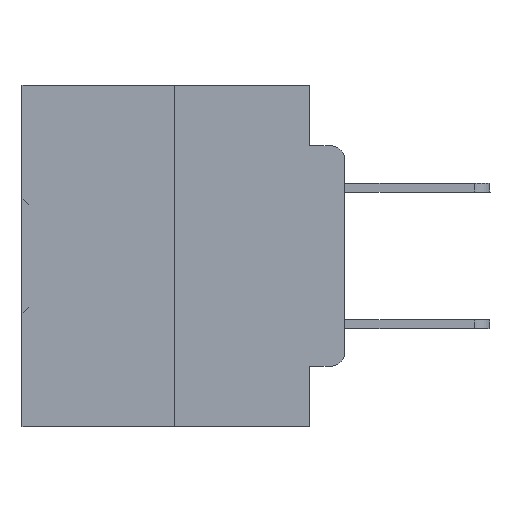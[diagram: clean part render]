
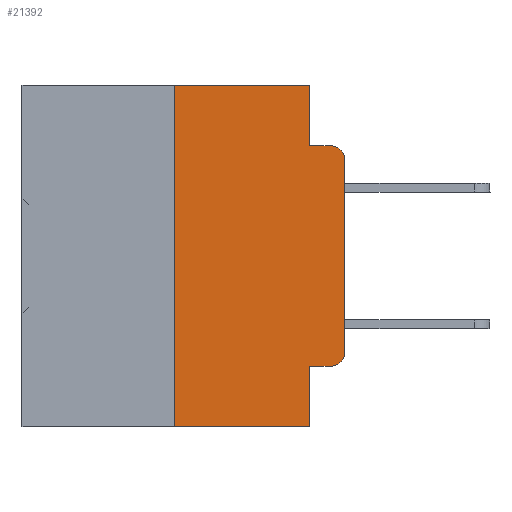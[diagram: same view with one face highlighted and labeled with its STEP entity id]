
A CAD part, left-side view. The second image highlights one B-rep face of the part: STEP entity #21392.
In plain terms, the highlighted planar face has unit normal (-1, 0, 0).
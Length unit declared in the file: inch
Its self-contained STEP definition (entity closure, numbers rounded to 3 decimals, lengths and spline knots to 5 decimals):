
#1253 = AXIS2_PLACEMENT_3D ( 'NONE', #6775, #26557, #9620 ) ;
#1346 = ORIENTED_EDGE ( 'NONE', *, *, #23523, .F. ) ;
#1879 = CARTESIAN_POINT ( 'NONE',  ( 0., 0.051, -0.4115 ) ) ;
#2084 = DIRECTION ( 'NONE',  ( 0., 0., -1. ) ) ;
#2875 = VECTOR ( 'NONE', #15385, 39.37008 ) ;
#3985 = CARTESIAN_POINT ( 'NONE',  ( 0., 0.051, 0. ) ) ;
#4234 = DIRECTION ( 'NONE',  ( 0., 0., 1. ) ) ;
#4539 = VERTEX_POINT ( 'NONE', #21378 ) ;
#4730 = CARTESIAN_POINT ( 'NONE',  ( 0., 0.25, -0.5 ) ) ;
#4980 = ORIENTED_EDGE ( 'NONE', *, *, #17506, .T. ) ;
#5742 = VECTOR ( 'NONE', #13150, 39.37008 ) ;
#6094 = VERTEX_POINT ( 'NONE', #4730 ) ;
#6095 = VECTOR ( 'NONE', #30946, 39.37008 ) ;
#6140 = DIRECTION ( 'NONE',  ( 0., 0., -1. ) ) ;
#6775 = CARTESIAN_POINT ( 'NONE',  ( 0., 0.02, -0.1085 ) ) ;
#7444 = CARTESIAN_POINT ( 'NONE',  ( 0., 0.051, -0.4115 ) ) ;
#7494 = CARTESIAN_POINT ( 'NONE',  ( 0., 0.473, -0.5 ) ) ;
#9620 = DIRECTION ( 'NONE',  ( 0., 0., -1. ) ) ;
#9769 = CARTESIAN_POINT ( 'NONE',  ( 0., 0.051, 0. ) ) ;
#10288 = ORIENTED_EDGE ( 'NONE', *, *, #15849, .T. ) ;
#10762 = ORIENTED_EDGE ( 'NONE', *, *, #18948, .F. ) ;
#11372 = AXIS2_PLACEMENT_3D ( 'NONE', #31407, #23121, #6140 ) ;
#11918 = AXIS2_PLACEMENT_3D ( 'NONE', #35868, #19095, #2084 ) ;
#11961 = VERTEX_POINT ( 'NONE', #1879 ) ;
#12064 = CARTESIAN_POINT ( 'NONE',  ( 0., 0., -0.3915 ) ) ;
#13150 = DIRECTION ( 'NONE',  ( 0., -1., 0. ) ) ;
#13276 = LINE ( 'NONE', #7444, #5742 ) ;
#13991 = EDGE_CURVE ( 'NONE', #31617, #19592, #15132, .T. ) ;
#14046 = CARTESIAN_POINT ( 'NONE',  ( 0., 0., 0. ) ) ;
#14082 = ORIENTED_EDGE ( 'NONE', *, *, #17052, .T. ) ;
#14471 = LINE ( 'NONE', #14046, #6095 ) ;
#14996 = CARTESIAN_POINT ( 'NONE',  ( 0., 0.02, -0.4115 ) ) ;
#15009 = LINE ( 'NONE', #24076, #36550 ) ;
#15132 = CIRCLE ( 'NONE', #11918, 0.02 ) ;
#15305 = LINE ( 'NONE', #7494, #30333 ) ;
#15385 = DIRECTION ( 'NONE',  ( 0., 0., -1. ) ) ;
#15725 = VERTEX_POINT ( 'NONE', #32226 ) ;
#15775 = VERTEX_POINT ( 'NONE', #35252 ) ;
#15849 = EDGE_CURVE ( 'NONE', #11961, #31617, #13276, .T. ) ;
#16867 = ORIENTED_EDGE ( 'NONE', *, *, #19712, .F. ) ;
#16913 = CARTESIAN_POINT ( 'NONE',  ( 0., 0.051, -0.0885 ) ) ;
#17024 = VECTOR ( 'NONE', #30952, 39.37008 ) ;
#17052 = EDGE_CURVE ( 'NONE', #19592, #15725, #14471, .T. ) ;
#17452 = EDGE_LOOP ( 'NONE', ( #14082, #23659, #26232, #1346, #10762, #18244, #4980, #16867, #10288, #24929 ) ) ;
#17506 = EDGE_CURVE ( 'NONE', #6094, #18776, #15305, .T. ) ;
#17936 = LINE ( 'NONE', #9769, #2875 ) ;
#18048 = CIRCLE ( 'NONE', #1253, 0.02 ) ;
#18094 = DIRECTION ( 'NONE',  ( 0., 0., -1. ) ) ;
#18244 = ORIENTED_EDGE ( 'NONE', *, *, #21614, .F. ) ;
#18776 = VERTEX_POINT ( 'NONE', #24757 ) ;
#18948 = EDGE_CURVE ( 'NONE', #20562, #27828, #24624, .T. ) ;
#19095 = DIRECTION ( 'NONE',  ( -1., 0., 0. ) ) ;
#19592 = VERTEX_POINT ( 'NONE', #12064 ) ;
#19712 = EDGE_CURVE ( 'NONE', #11961, #18776, #22371, .T. ) ;
#19796 = DIRECTION ( 'NONE',  ( 0., -1., 0. ) ) ;
#19875 = LINE ( 'NONE', #16913, #34764 ) ;
#20562 = VERTEX_POINT ( 'NONE', #33514 ) ;
#21378 = CARTESIAN_POINT ( 'NONE',  ( 0., 0.02, -0.0885 ) ) ;
#21392 = ADVANCED_FACE ( 'NONE', ( #35755 ), #34202, .F. ) ;
#21614 = EDGE_CURVE ( 'NONE', #6094, #20562, #15009, .T. ) ;
#22371 = LINE ( 'NONE', #3985, #36302 ) ;
#22524 = CARTESIAN_POINT ( 'NONE',  ( 0., 0.051, 0. ) ) ;
#23121 = DIRECTION ( 'NONE',  ( 1., 0., 0. ) ) ;
#23523 = EDGE_CURVE ( 'NONE', #27828, #15775, #17936, .T. ) ;
#23659 = ORIENTED_EDGE ( 'NONE', *, *, #28441, .T. ) ;
#24076 = CARTESIAN_POINT ( 'NONE',  ( 0., 0.25, 0. ) ) ;
#24624 = LINE ( 'NONE', #25365, #17024 ) ;
#24757 = CARTESIAN_POINT ( 'NONE',  ( 0., 0.051, -0.5 ) ) ;
#24929 = ORIENTED_EDGE ( 'NONE', *, *, #13991, .T. ) ;
#25365 = CARTESIAN_POINT ( 'NONE',  ( 0., 0.473, 0. ) ) ;
#26232 = ORIENTED_EDGE ( 'NONE', *, *, #27253, .F. ) ;
#26557 = DIRECTION ( 'NONE',  ( -1., 0., 0. ) ) ;
#27253 = EDGE_CURVE ( 'NONE', #15775, #4539, #19875, .T. ) ;
#27828 = VERTEX_POINT ( 'NONE', #22524 ) ;
#28441 = EDGE_CURVE ( 'NONE', #15725, #4539, #18048, .T. ) ;
#30333 = VECTOR ( 'NONE', #32851, 39.37008 ) ;
#30946 = DIRECTION ( 'NONE',  ( 0., 0., 1. ) ) ;
#30952 = DIRECTION ( 'NONE',  ( 0., -1., 0. ) ) ;
#31407 = CARTESIAN_POINT ( 'NONE',  ( 0., 0.473, 0. ) ) ;
#31617 = VERTEX_POINT ( 'NONE', #14996 ) ;
#32226 = CARTESIAN_POINT ( 'NONE',  ( 0., 0., -0.1085 ) ) ;
#32851 = DIRECTION ( 'NONE',  ( 0., -1., 0. ) ) ;
#33514 = CARTESIAN_POINT ( 'NONE',  ( 0., 0.25, 0. ) ) ;
#34202 = PLANE ( 'NONE',  #11372 ) ;
#34764 = VECTOR ( 'NONE', #19796, 39.37008 ) ;
#35252 = CARTESIAN_POINT ( 'NONE',  ( 0., 0.051, -0.0885 ) ) ;
#35755 = FACE_OUTER_BOUND ( 'NONE', #17452, .T. ) ;
#35868 = CARTESIAN_POINT ( 'NONE',  ( 0., 0.02, -0.3915 ) ) ;
#36302 = VECTOR ( 'NONE', #18094, 39.37008 ) ;
#36550 = VECTOR ( 'NONE', #4234, 39.37008 ) ;
